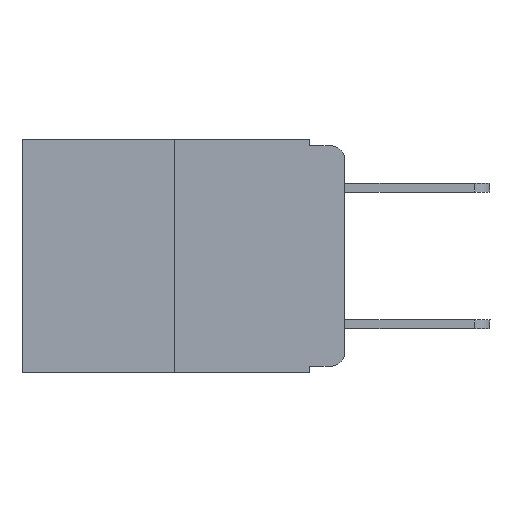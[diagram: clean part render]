
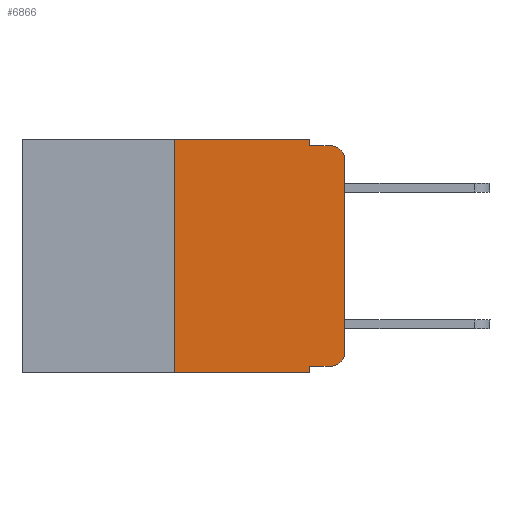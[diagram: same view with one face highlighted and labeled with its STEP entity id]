
A CAD part, left-side view. The second image highlights one B-rep face of the part: STEP entity #6866.
In plain terms, the highlighted planar face has unit normal (-1, 0, 0).
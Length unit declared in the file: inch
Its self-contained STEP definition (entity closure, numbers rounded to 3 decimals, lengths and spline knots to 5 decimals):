
#24 = ORIENTED_EDGE ( 'NONE', *, *, #14636, .T. ) ;
#205 = ORIENTED_EDGE ( 'NONE', *, *, #6972, .T. ) ;
#245 = CARTESIAN_POINT ( 'NONE',  ( 0., 0.051, -0.343 ) ) ;
#270 = ORIENTED_EDGE ( 'NONE', *, *, #478, .T. ) ;
#478 = EDGE_CURVE ( 'NONE', #16834, #7942, #5647, .T. ) ;
#488 = CARTESIAN_POINT ( 'NONE',  ( 0., 0.02, -0.03 ) ) ;
#511 = ORIENTED_EDGE ( 'NONE', *, *, #1376, .T. ) ;
#565 = LINE ( 'NONE', #5680, #13719 ) ;
#574 = EDGE_CURVE ( 'NONE', #2749, #12193, #9955, .T. ) ;
#859 = EDGE_CURVE ( 'NONE', #13649, #2749, #13138, .T. ) ;
#1067 = CARTESIAN_POINT ( 'NONE',  ( 0., 0.473, 0. ) ) ;
#1251 = DIRECTION ( 'NONE',  ( 0., -1., 0. ) ) ;
#1257 = CARTESIAN_POINT ( 'NONE',  ( 0., 0.25, -0.343 ) ) ;
#1376 = EDGE_CURVE ( 'NONE', #7942, #17046, #7629, .T. ) ;
#1709 = CARTESIAN_POINT ( 'NONE',  ( 0., 0.051, 0. ) ) ;
#1779 = DIRECTION ( 'NONE',  ( 0., -1., 0. ) ) ;
#1898 = DIRECTION ( 'NONE',  ( 0., 0., 1. ) ) ;
#2003 = ORIENTED_EDGE ( 'NONE', *, *, #13034, .T. ) ;
#2137 = CARTESIAN_POINT ( 'NONE',  ( 0., 0.25, 0. ) ) ;
#2749 = VERTEX_POINT ( 'NONE', #1709 ) ;
#2890 = CARTESIAN_POINT ( 'NONE',  ( 0., 0., -0.03 ) ) ;
#3039 = DIRECTION ( 'NONE',  ( 0., 0., -1. ) ) ;
#3104 = EDGE_CURVE ( 'NONE', #12193, #8828, #4338, .T. ) ;
#3340 = CARTESIAN_POINT ( 'NONE',  ( 0., 0.02, -0.333 ) ) ;
#3675 = VECTOR ( 'NONE', #14609, 39.37008 ) ;
#4270 = EDGE_LOOP ( 'NONE', ( #24, #2003, #16617, #10089, #11464, #7128, #205, #9343, #270, #511 ) ) ;
#4338 = LINE ( 'NONE', #13840, #14977 ) ;
#5647 = LINE ( 'NONE', #11008, #13963 ) ;
#5680 = CARTESIAN_POINT ( 'NONE',  ( 0., 0.25, 0. ) ) ;
#5737 = CARTESIAN_POINT ( 'NONE',  ( 0., 0.051, 0. ) ) ;
#6756 = CARTESIAN_POINT ( 'NONE',  ( 0., 0.473, -0.343 ) ) ;
#6866 = ADVANCED_FACE ( 'NONE', ( #10707 ), #15933, .F. ) ;
#6901 = DIRECTION ( 'NONE',  ( -1., 0., 0. ) ) ;
#6972 = EDGE_CURVE ( 'NONE', #9099, #9559, #13459, .T. ) ;
#7075 = CARTESIAN_POINT ( 'NONE',  ( 0., 0.02, -0.313 ) ) ;
#7128 = ORIENTED_EDGE ( 'NONE', *, *, #17019, .F. ) ;
#7581 = DIRECTION ( 'NONE',  ( 0., -1., 0. ) ) ;
#7629 = CIRCLE ( 'NONE', #8733, 0.02 ) ;
#7821 = CARTESIAN_POINT ( 'NONE',  ( 0., 0., 0. ) ) ;
#7942 = VERTEX_POINT ( 'NONE', #3340 ) ;
#8234 = CARTESIAN_POINT ( 'NONE',  ( 0., 0., -0.313 ) ) ;
#8334 = VECTOR ( 'NONE', #11872, 39.37008 ) ;
#8545 = DIRECTION ( 'NONE',  ( 0., 0., -1. ) ) ;
#8733 = AXIS2_PLACEMENT_3D ( 'NONE', #7075, #6901, #3039 ) ;
#8828 = VERTEX_POINT ( 'NONE', #10069 ) ;
#8962 = CARTESIAN_POINT ( 'NONE',  ( 0., 0.051, 0. ) ) ;
#9099 = VERTEX_POINT ( 'NONE', #1257 ) ;
#9343 = ORIENTED_EDGE ( 'NONE', *, *, #14533, .F. ) ;
#9559 = VERTEX_POINT ( 'NONE', #245 ) ;
#9621 = CARTESIAN_POINT ( 'NONE',  ( 0., 0.051, -0.01 ) ) ;
#9955 = LINE ( 'NONE', #5737, #17085 ) ;
#10069 = CARTESIAN_POINT ( 'NONE',  ( 0., 0.02, -0.01 ) ) ;
#10089 = ORIENTED_EDGE ( 'NONE', *, *, #574, .F. ) ;
#10367 = LINE ( 'NONE', #7821, #8334 ) ;
#10628 = DIRECTION ( 'NONE',  ( 0., 0., -1. ) ) ;
#10707 = FACE_OUTER_BOUND ( 'NONE', #4270, .T. ) ;
#11008 = CARTESIAN_POINT ( 'NONE',  ( 0., 0.051, -0.333 ) ) ;
#11113 = VERTEX_POINT ( 'NONE', #2890 ) ;
#11138 = DIRECTION ( 'NONE',  ( -1., 0., 0. ) ) ;
#11245 = LINE ( 'NONE', #8962, #14519 ) ;
#11464 = ORIENTED_EDGE ( 'NONE', *, *, #859, .F. ) ;
#11640 = AXIS2_PLACEMENT_3D ( 'NONE', #16098, #16184, #10628 ) ;
#11872 = DIRECTION ( 'NONE',  ( 0., 0., 1. ) ) ;
#12193 = VERTEX_POINT ( 'NONE', #9621 ) ;
#12646 = VECTOR ( 'NONE', #7581, 39.37008 ) ;
#13034 = EDGE_CURVE ( 'NONE', #11113, #8828, #16457, .T. ) ;
#13138 = LINE ( 'NONE', #1067, #12646 ) ;
#13191 = CARTESIAN_POINT ( 'NONE',  ( 0., 0.051, -0.333 ) ) ;
#13459 = LINE ( 'NONE', #6756, #3675 ) ;
#13649 = VERTEX_POINT ( 'NONE', #2137 ) ;
#13719 = VECTOR ( 'NONE', #1898, 39.37008 ) ;
#13840 = CARTESIAN_POINT ( 'NONE',  ( 0., 0.051, -0.01 ) ) ;
#13963 = VECTOR ( 'NONE', #1251, 39.37008 ) ;
#14519 = VECTOR ( 'NONE', #16726, 39.37008 ) ;
#14533 = EDGE_CURVE ( 'NONE', #16834, #9559, #11245, .T. ) ;
#14609 = DIRECTION ( 'NONE',  ( 0., -1., 0. ) ) ;
#14636 = EDGE_CURVE ( 'NONE', #17046, #11113, #10367, .T. ) ;
#14977 = VECTOR ( 'NONE', #1779, 39.37008 ) ;
#15121 = DIRECTION ( 'NONE',  ( 0., 0., -1. ) ) ;
#15886 = AXIS2_PLACEMENT_3D ( 'NONE', #488, #11138, #15121 ) ;
#15933 = PLANE ( 'NONE',  #11640 ) ;
#16098 = CARTESIAN_POINT ( 'NONE',  ( 0., 0.473, 0. ) ) ;
#16184 = DIRECTION ( 'NONE',  ( 1., 0., 0. ) ) ;
#16457 = CIRCLE ( 'NONE', #15886, 0.02 ) ;
#16617 = ORIENTED_EDGE ( 'NONE', *, *, #3104, .F. ) ;
#16726 = DIRECTION ( 'NONE',  ( 0., 0., -1. ) ) ;
#16834 = VERTEX_POINT ( 'NONE', #13191 ) ;
#17019 = EDGE_CURVE ( 'NONE', #9099, #13649, #565, .T. ) ;
#17046 = VERTEX_POINT ( 'NONE', #8234 ) ;
#17085 = VECTOR ( 'NONE', #8545, 39.37008 ) ;
